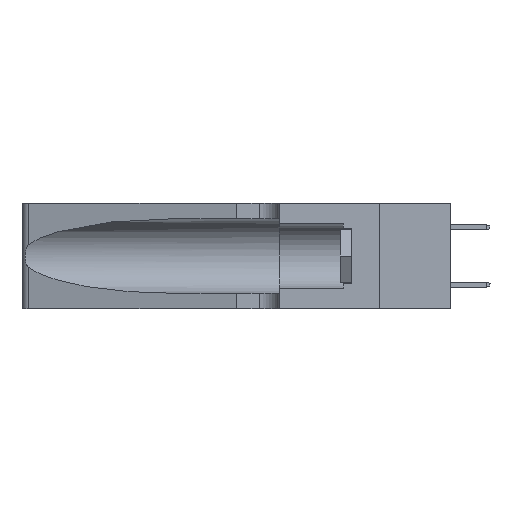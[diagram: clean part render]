
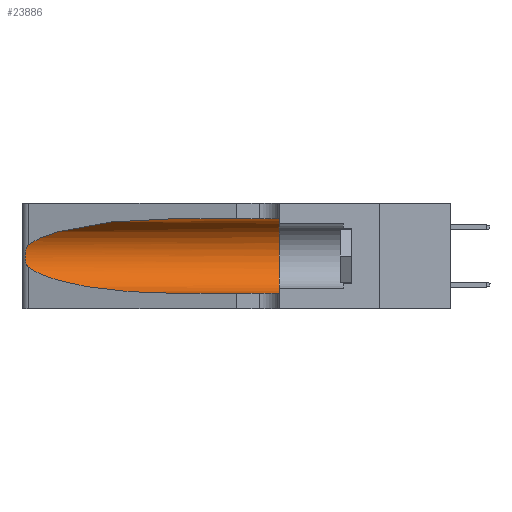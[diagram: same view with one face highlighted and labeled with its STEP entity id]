
A CAD part, left-side view. The second image highlights one B-rep face of the part: STEP entity #23886.
In plain terms, the highlighted cylindrical face has radius 3.308 mm (diameter 6.617 mm), a partial arc.
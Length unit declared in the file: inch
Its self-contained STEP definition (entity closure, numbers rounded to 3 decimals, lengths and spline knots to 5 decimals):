
#171 = DIRECTION ( 'NONE',  ( 0., 1., 0. ) ) ;
#383 = CARTESIAN_POINT ( 'NONE',  ( 0.1305, 0.35, 0.31525 ) ) ;
#1507 = CARTESIAN_POINT ( 'NONE',  ( 0.25639, 1.23184, 0.21858 ) ) ;
#1826 = EDGE_CURVE ( 'NONE', #13587, #20117, #10801, .T. ) ;
#2031 = VECTOR ( 'NONE', #2760, 39.37008 ) ;
#2036 = DIRECTION ( 'NONE',  ( 0., -1., 0. ) ) ;
#2161 = CARTESIAN_POINT ( 'NONE',  ( 0.18966, 0.96281, 0.05475 ) ) ;
#2760 = DIRECTION ( 'NONE',  ( 0., -1., 0. ) ) ;
#3761 = CARTESIAN_POINT ( 'NONE',  ( 0.25789, 1.23486, 0.15765 ) ) ;
#4259 = CARTESIAN_POINT ( 'NONE',  ( 0.25555, 1.22993, 0.14849 ) ) ;
#5269 =( BOUNDED_CURVE ( )  B_SPLINE_CURVE ( 3, ( #31181, #17788, #2161, #23097 ),
 .UNSPECIFIED., .F., .F. ) 
 B_SPLINE_CURVE_WITH_KNOTS ( ( 4, 4 ),
 ( 3.44316, 4.71239 ),
 .UNSPECIFIED. ) 
 CURVE ( )  GEOMETRIC_REPRESENTATION_ITEM ( )  RATIONAL_B_SPLINE_CURVE ( ( 1., 0.87, 0.87, 1. ) ) 
 REPRESENTATION_ITEM ( '' )  );
#5555 = CARTESIAN_POINT ( 'NONE',  ( 0.25487, 1.22718, 0.22369 ) ) ;
#5674 = CARTESIAN_POINT ( 'NONE',  ( 0.1305, 0.35, 0.185 ) ) ;
#6448 = DIRECTION ( 'NONE',  ( 0., -1., 0. ) ) ;
#7015 = FACE_OUTER_BOUND ( 'NONE', #29669, .T. ) ;
#7105 = EDGE_CURVE ( 'NONE', #26421, #13054, #22406, .T. ) ;
#8147 = ORIENTED_EDGE ( 'NONE', *, *, #23572, .F. ) ;
#8370 = ORIENTED_EDGE ( 'NONE', *, *, #1826, .T. ) ;
#8901 = CARTESIAN_POINT ( 'NONE',  ( 0.25639, 1.23186, 0.15144 ) ) ;
#9409 = CARTESIAN_POINT ( 'NONE',  ( 0.26075, 1.23896, 0.19203 ) ) ;
#10679 = EDGE_CURVE ( 'NONE', #20117, #18286, #27965, .T. ) ;
#10801 =( BOUNDED_CURVE ( )  B_SPLINE_CURVE ( 3, ( #19085, #16017, #29557, #16182 ),
 .UNSPECIFIED., .F., .T. ) 
 B_SPLINE_CURVE_WITH_KNOTS ( ( 4, 4 ),
 ( 1.5708, 2.84003 ),
 .UNSPECIFIED. ) 
 CURVE ( )  GEOMETRIC_REPRESENTATION_ITEM ( )  RATIONAL_B_SPLINE_CURVE ( ( 1., 0.87, 0.87, 1. ) ) 
 REPRESENTATION_ITEM ( '' )  );
#11889 = ORIENTED_EDGE ( 'NONE', *, *, #7105, .T. ) ;
#12138 = CARTESIAN_POINT ( 'NONE',  ( 0.1305, 0.72297, 0.05475 ) ) ;
#12188 = DIRECTION ( 'NONE',  ( 0., 0., -1. ) ) ;
#13054 = VERTEX_POINT ( 'NONE', #28023 ) ;
#13587 = VERTEX_POINT ( 'NONE', #27542 ) ;
#13657 = CIRCLE ( 'NONE', #24585, 0.13025 ) ;
#14585 = CARTESIAN_POINT ( 'NONE',  ( 0.1305, 1.61858, 0.185 ) ) ;
#14737 = CARTESIAN_POINT ( 'NONE',  ( 0.25487, 1.22718, 0.14631 ) ) ;
#16017 = CARTESIAN_POINT ( 'NONE',  ( 0.18966, 0.96281, 0.31525 ) ) ;
#16182 = CARTESIAN_POINT ( 'NONE',  ( 0.25487, 1.22718, 0.22369 ) ) ;
#17302 = CARTESIAN_POINT ( 'NONE',  ( 0.26017, 1.23833, 0.17102 ) ) ;
#17788 = CARTESIAN_POINT ( 'NONE',  ( 0.2373, 1.15595, 0.08982 ) ) ;
#18286 = VERTEX_POINT ( 'NONE', #26022 ) ;
#19085 = CARTESIAN_POINT ( 'NONE',  ( 0.1305, 0.72297, 0.31525 ) ) ;
#19190 = VECTOR ( 'NONE', #6448, 39.37008 ) ;
#20117 = VERTEX_POINT ( 'NONE', #5555 ) ;
#21699 = EDGE_CURVE ( 'NONE', #13587, #32510, #23867, .T. ) ;
#22072 = CARTESIAN_POINT ( 'NONE',  ( 0.1305, 1.61858, 0.05475 ) ) ;
#22406 = LINE ( 'NONE', #22072, #19190 ) ;
#22418 = EDGE_CURVE ( 'NONE', #18286, #26421, #5269, .T. ) ;
#22454 = CARTESIAN_POINT ( 'NONE',  ( 0.25787, 1.23484, 0.2124 ) ) ;
#22619 = CARTESIAN_POINT ( 'NONE',  ( 0.25856, 1.23593, 0.16098 ) ) ;
#23097 = CARTESIAN_POINT ( 'NONE',  ( 0.1305, 0.72297, 0.05475 ) ) ;
#23572 = EDGE_CURVE ( 'NONE', #32510, #13054, #13657, .T. ) ;
#23867 = LINE ( 'NONE', #24042, #2031 ) ;
#23886 = ADVANCED_FACE ( 'NONE', ( #7015 ), #25551, .F. ) ;
#24042 = CARTESIAN_POINT ( 'NONE',  ( 0.1305, 1.61858, 0.31525 ) ) ;
#24585 = AXIS2_PLACEMENT_3D ( 'NONE', #5674, #171, #26439 ) ;
#25551 = CYLINDRICAL_SURFACE ( 'NONE', #32835, 0.13025 ) ;
#26022 = CARTESIAN_POINT ( 'NONE',  ( 0.25487, 1.22718, 0.14631 ) ) ;
#26421 = VERTEX_POINT ( 'NONE', #12138 ) ;
#26439 = DIRECTION ( 'NONE',  ( 0., 0., 1. ) ) ;
#26461 = ORIENTED_EDGE ( 'NONE', *, *, #22418, .T. ) ;
#27064 = ORIENTED_EDGE ( 'NONE', *, *, #21699, .F. ) ;
#27542 = CARTESIAN_POINT ( 'NONE',  ( 0.1305, 0.72297, 0.31525 ) ) ;
#27767 = CARTESIAN_POINT ( 'NONE',  ( 0.26018, 1.23835, 0.19895 ) ) ;
#27965 = B_SPLINE_CURVE_WITH_KNOTS ( 'NONE', 3,
 ( #32754, #30174, #1507, #22454, #32918, #27767, #9409, #32417, #17302, #22619, #3761, #8901, #4259, #14737 ),
 .UNSPECIFIED., .F., .F.,
 ( 4, 2, 2, 2, 2, 2, 4 ),
 ( 0., 0.00027, 0.00053, 0.00107, 0.0016, 0.00187, 0.00214 ),
 .UNSPECIFIED. ) ;
#28023 = CARTESIAN_POINT ( 'NONE',  ( 0.1305, 0.35, 0.05475 ) ) ;
#29557 = CARTESIAN_POINT ( 'NONE',  ( 0.2373, 1.15595, 0.28018 ) ) ;
#29669 = EDGE_LOOP ( 'NONE', ( #8370, #33682, #26461, #11889, #8147, #27064 ) ) ;
#30174 = CARTESIAN_POINT ( 'NONE',  ( 0.25555, 1.22994, 0.2215 ) ) ;
#31181 = CARTESIAN_POINT ( 'NONE',  ( 0.25487, 1.22718, 0.14631 ) ) ;
#32417 = CARTESIAN_POINT ( 'NONE',  ( 0.26075, 1.23896, 0.178 ) ) ;
#32510 = VERTEX_POINT ( 'NONE', #383 ) ;
#32754 = CARTESIAN_POINT ( 'NONE',  ( 0.25487, 1.22718, 0.22369 ) ) ;
#32835 = AXIS2_PLACEMENT_3D ( 'NONE', #14585, #2036, #12188 ) ;
#32918 = CARTESIAN_POINT ( 'NONE',  ( 0.25854, 1.2359, 0.20912 ) ) ;
#33682 = ORIENTED_EDGE ( 'NONE', *, *, #10679, .T. ) ;
